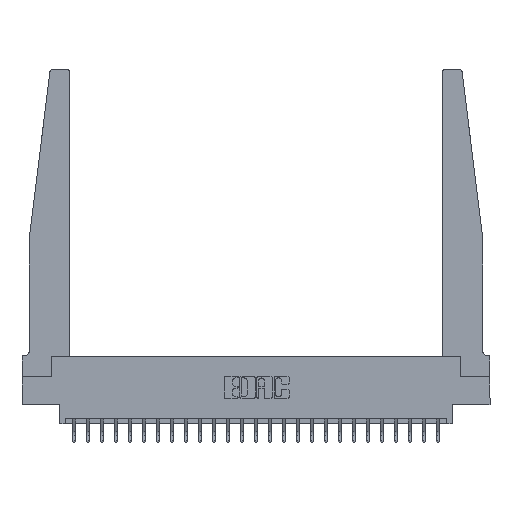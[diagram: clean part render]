
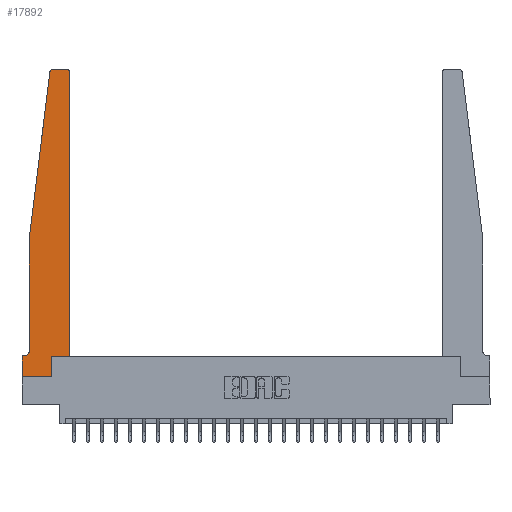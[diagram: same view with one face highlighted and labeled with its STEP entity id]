
A CAD part, top view. The second image highlights one B-rep face of the part: STEP entity #17892.
In plain terms, the highlighted planar face has unit normal (0, 0, 1).
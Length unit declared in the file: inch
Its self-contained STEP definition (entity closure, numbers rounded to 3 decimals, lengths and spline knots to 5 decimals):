
#150 = EDGE_CURVE ( 'NONE', #6796, #15961, #22341, .T. ) ;
#377 = VERTEX_POINT ( 'NONE', #13134 ) ;
#726 = EDGE_CURVE ( 'NONE', #7480, #6796, #5247, .T. ) ;
#730 = CARTESIAN_POINT ( 'NONE',  ( 0.24675, 2.72367, 0.37 ) ) ;
#959 = DIRECTION ( 'NONE',  ( -0.122, -0.992, 0. ) ) ;
#1041 = VERTEX_POINT ( 'NONE', #10795 ) ;
#1238 = VERTEX_POINT ( 'NONE', #17617 ) ;
#1665 = CARTESIAN_POINT ( 'NONE',  ( 0.25, 2.75, 0.37 ) ) ;
#1669 = DIRECTION ( 'NONE',  ( 0., 1., 0. ) ) ;
#1777 = CARTESIAN_POINT ( 'NONE',  ( 0.015, 0.2375, 0.37 ) ) ;
#1915 = DIRECTION ( 'NONE',  ( -1., 0., 0. ) ) ;
#2052 = ORIENTED_EDGE ( 'NONE', *, *, #4473, .T. ) ;
#2092 = ORIENTED_EDGE ( 'NONE', *, *, #12545, .T. ) ;
#2421 = CARTESIAN_POINT ( 'NONE',  ( 0.015, 0.1875, 0.37 ) ) ;
#2686 = VECTOR ( 'NONE', #8580, 39.37008 ) ;
#2782 = EDGE_CURVE ( 'NONE', #377, #9838, #5514, .T. ) ;
#2862 = ORIENTED_EDGE ( 'NONE', *, *, #6697, .T. ) ;
#3078 = ORIENTED_EDGE ( 'NONE', *, *, #14747, .T. ) ;
#3116 = DIRECTION ( 'NONE',  ( 0., -1., 0. ) ) ;
#3154 = CARTESIAN_POINT ( 'NONE',  ( 0., 0., 0.37 ) ) ;
#3274 = LINE ( 'NONE', #3154, #23427 ) ;
#3371 = FACE_OUTER_BOUND ( 'NONE', #11177, .T. ) ;
#3606 = LINE ( 'NONE', #1665, #11249 ) ;
#3734 = AXIS2_PLACEMENT_3D ( 'NONE', #21620, #6323, #17792 ) ;
#3742 = CARTESIAN_POINT ( 'NONE',  ( 0., 0.1875, 0.37 ) ) ;
#3950 = ORIENTED_EDGE ( 'NONE', *, *, #11265, .T. ) ;
#4212 = CARTESIAN_POINT ( 'NONE',  ( 0.065, 1.25, 0.37 ) ) ;
#4276 = VECTOR ( 'NONE', #12994, 39.37008 ) ;
#4473 = EDGE_CURVE ( 'NONE', #23612, #18694, #24619, .T. ) ;
#4671 = DIRECTION ( 'NONE',  ( -1., 0., 0. ) ) ;
#4727 = ORIENTED_EDGE ( 'NONE', *, *, #14360, .T. ) ;
#4824 = LINE ( 'NONE', #12699, #13325 ) ;
#5040 = LINE ( 'NONE', #22096, #2686 ) ;
#5247 = LINE ( 'NONE', #7367, #4276 ) ;
#5335 = DIRECTION ( 'NONE',  ( 1., 0., 0. ) ) ;
#5514 = LINE ( 'NONE', #7658, #21881 ) ;
#6323 = DIRECTION ( 'NONE',  ( 0., 0., 1. ) ) ;
#6398 = DIRECTION ( 'NONE',  ( 0., 0., 1. ) ) ;
#6409 = VERTEX_POINT ( 'NONE', #11412 ) ;
#6697 = EDGE_CURVE ( 'NONE', #1238, #1041, #5040, .T. ) ;
#6796 = VERTEX_POINT ( 'NONE', #3742 ) ;
#6934 = DIRECTION ( 'NONE',  ( 0., -1., 0. ) ) ;
#7089 = EDGE_CURVE ( 'NONE', #6409, #7867, #9207, .T. ) ;
#7367 = CARTESIAN_POINT ( 'NONE',  ( 0.065, 0.1875, 0.37 ) ) ;
#7480 = VERTEX_POINT ( 'NONE', #2421 ) ;
#7658 = CARTESIAN_POINT ( 'NONE',  ( 0.425, 0.18, 0.37 ) ) ;
#7867 = VERTEX_POINT ( 'NONE', #730 ) ;
#7908 = VERTEX_POINT ( 'NONE', #10413 ) ;
#8580 = DIRECTION ( 'NONE',  ( 0., 1., 0. ) ) ;
#9207 = CIRCLE ( 'NONE', #19788, 0.03 ) ;
#9265 = CARTESIAN_POINT ( 'NONE',  ( 0.425, 0.18, 0.37 ) ) ;
#9342 = ORIENTED_EDGE ( 'NONE', *, *, #24731, .T. ) ;
#9809 = EDGE_CURVE ( 'NONE', #1041, #377, #22784, .T. ) ;
#9838 = VERTEX_POINT ( 'NONE', #15497 ) ;
#10212 = CIRCLE ( 'NONE', #13430, 0.05 ) ;
#10413 = CARTESIAN_POINT ( 'NONE',  ( 0.395, 2.75, 0.37 ) ) ;
#10795 = CARTESIAN_POINT ( 'NONE',  ( 0.2605, 0.18, 0.37 ) ) ;
#11139 = DIRECTION ( 'NONE',  ( 1., 0., 0. ) ) ;
#11177 = EDGE_LOOP ( 'NONE', ( #9342, #15170, #3950, #2052, #2092, #25121, #24341, #3078, #2862, #13482, #14614, #4727 ) ) ;
#11249 = VECTOR ( 'NONE', #4671, 39.37008 ) ;
#11265 = EDGE_CURVE ( 'NONE', #7867, #23612, #4824, .T. ) ;
#11412 = CARTESIAN_POINT ( 'NONE',  ( 0.27653, 2.75, 0.37 ) ) ;
#11469 = DIRECTION ( 'NONE',  ( 0., 0., -1. ) ) ;
#12291 = AXIS2_PLACEMENT_3D ( 'NONE', #21081, #13157, #22852 ) ;
#12545 = EDGE_CURVE ( 'NONE', #18694, #7480, #10212, .T. ) ;
#12699 = CARTESIAN_POINT ( 'NONE',  ( 0.065, 1.25, 0.37 ) ) ;
#12908 = CARTESIAN_POINT ( 'NONE',  ( 0.065, 1.25, 0.37 ) ) ;
#12994 = DIRECTION ( 'NONE',  ( -1., 0., 0. ) ) ;
#13134 = CARTESIAN_POINT ( 'NONE',  ( 0.425, 0.18, 0.37 ) ) ;
#13157 = DIRECTION ( 'NONE',  ( 0., 0., 1. ) ) ;
#13325 = VECTOR ( 'NONE', #959, 39.37008 ) ;
#13430 = AXIS2_PLACEMENT_3D ( 'NONE', #1777, #11469, #1915 ) ;
#13482 = ORIENTED_EDGE ( 'NONE', *, *, #9809, .T. ) ;
#14360 = EDGE_CURVE ( 'NONE', #9838, #7908, #24472, .T. ) ;
#14614 = ORIENTED_EDGE ( 'NONE', *, *, #2782, .T. ) ;
#14747 = EDGE_CURVE ( 'NONE', #15961, #1238, #3274, .T. ) ;
#15075 = PLANE ( 'NONE',  #12291 ) ;
#15170 = ORIENTED_EDGE ( 'NONE', *, *, #7089, .T. ) ;
#15497 = CARTESIAN_POINT ( 'NONE',  ( 0.425, 2.72, 0.37 ) ) ;
#15961 = VERTEX_POINT ( 'NONE', #20611 ) ;
#16468 = CARTESIAN_POINT ( 'NONE',  ( 0.27653, 2.72, 0.37 ) ) ;
#17617 = CARTESIAN_POINT ( 'NONE',  ( 0.2605, 0., 0.37 ) ) ;
#17792 = DIRECTION ( 'NONE',  ( 1., 0., 0. ) ) ;
#17892 = ADVANCED_FACE ( 'NONE', ( #3371 ), #15075, .T. ) ;
#17893 = VECTOR ( 'NONE', #3116, 39.37008 ) ;
#18694 = VERTEX_POINT ( 'NONE', #22771 ) ;
#19772 = VECTOR ( 'NONE', #6934, 39.37008 ) ;
#19788 = AXIS2_PLACEMENT_3D ( 'NONE', #16468, #6398, #21946 ) ;
#20316 = CARTESIAN_POINT ( 'NONE',  ( 0., 0., 0.37 ) ) ;
#20611 = CARTESIAN_POINT ( 'NONE',  ( 0., 0., 0.37 ) ) ;
#21081 = CARTESIAN_POINT ( 'NONE',  ( 0., 0.1875, 0.37 ) ) ;
#21620 = CARTESIAN_POINT ( 'NONE',  ( 0.395, 2.72, 0.37 ) ) ;
#21881 = VECTOR ( 'NONE', #1669, 39.37008 ) ;
#21946 = DIRECTION ( 'NONE',  ( 1., 0., 0. ) ) ;
#22096 = CARTESIAN_POINT ( 'NONE',  ( 0.2605, 0.18, 0.37 ) ) ;
#22341 = LINE ( 'NONE', #20316, #19772 ) ;
#22771 = CARTESIAN_POINT ( 'NONE',  ( 0.065, 0.2375, 0.37 ) ) ;
#22784 = LINE ( 'NONE', #9265, #23356 ) ;
#22852 = DIRECTION ( 'NONE',  ( 1., 0., 0. ) ) ;
#23356 = VECTOR ( 'NONE', #5335, 39.37008 ) ;
#23427 = VECTOR ( 'NONE', #11139, 39.37008 ) ;
#23612 = VERTEX_POINT ( 'NONE', #4212 ) ;
#24341 = ORIENTED_EDGE ( 'NONE', *, *, #150, .T. ) ;
#24472 = CIRCLE ( 'NONE', #3734, 0.03 ) ;
#24619 = LINE ( 'NONE', #12908, #17893 ) ;
#24731 = EDGE_CURVE ( 'NONE', #7908, #6409, #3606, .T. ) ;
#25121 = ORIENTED_EDGE ( 'NONE', *, *, #726, .T. ) ;
